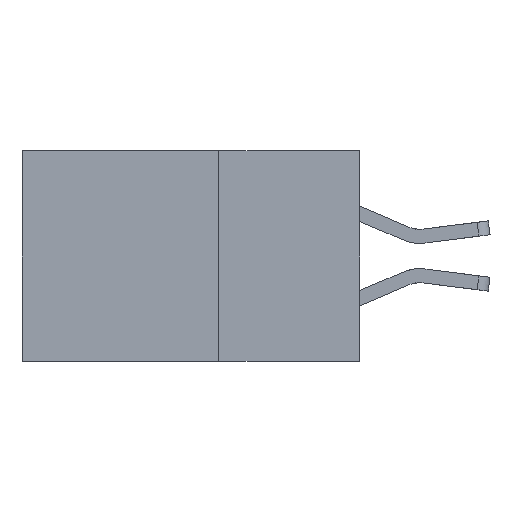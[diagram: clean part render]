
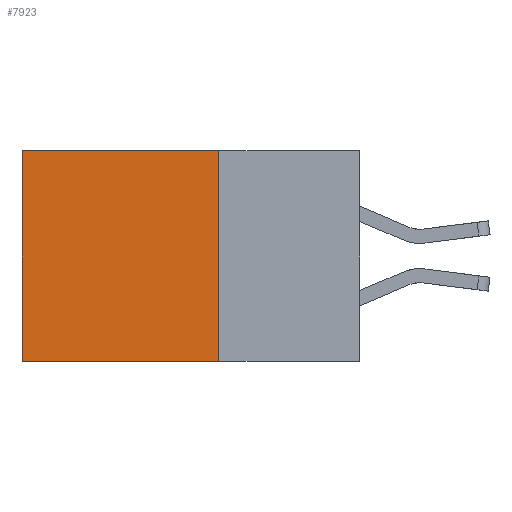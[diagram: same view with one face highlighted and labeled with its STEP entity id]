
A CAD part, left-side view. The second image highlights one B-rep face of the part: STEP entity #7923.
In plain terms, the highlighted planar face has unit normal (-1, 0, 0).
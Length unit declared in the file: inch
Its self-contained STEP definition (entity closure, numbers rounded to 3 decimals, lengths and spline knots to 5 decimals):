
#9 = ORIENTED_EDGE ( 'NONE', *, *, #3762, .F. ) ;
#280 = CARTESIAN_POINT ( 'NONE',  ( 0.2875, 0.25, -0.375 ) ) ;
#349 = CARTESIAN_POINT ( 'NONE',  ( 0.2875, 0.6, -0.375 ) ) ;
#648 = CARTESIAN_POINT ( 'NONE',  ( 0.2875, 0.25, 0. ) ) ;
#745 = VERTEX_POINT ( 'NONE', #4051 ) ;
#1106 = ORIENTED_EDGE ( 'NONE', *, *, #2413, .T. ) ;
#1216 = EDGE_CURVE ( 'NONE', #6039, #4882, #4200, .T. ) ;
#1244 = LINE ( 'NONE', #6938, #5781 ) ;
#1268 = EDGE_LOOP ( 'NONE', ( #1106, #9, #4151, #8144 ) ) ;
#1804 = VECTOR ( 'NONE', #7164, 39.37008 ) ;
#2143 = VECTOR ( 'NONE', #5949, 39.37008 ) ;
#2364 = LINE ( 'NONE', #8767, #2143 ) ;
#2413 = EDGE_CURVE ( 'NONE', #4882, #745, #3729, .T. ) ;
#2790 = CARTESIAN_POINT ( 'NONE',  ( 0.2875, 0.6, 0. ) ) ;
#3080 = DIRECTION ( 'NONE',  ( 1., 0., 0. ) ) ;
#3464 = VECTOR ( 'NONE', #7090, 39.37008 ) ;
#3669 = CARTESIAN_POINT ( 'NONE',  ( 0.2875, 0.25, 0. ) ) ;
#3729 = LINE ( 'NONE', #349, #1804 ) ;
#3762 = EDGE_CURVE ( 'NONE', #4008, #745, #1244, .T. ) ;
#4008 = VERTEX_POINT ( 'NONE', #280 ) ;
#4051 = CARTESIAN_POINT ( 'NONE',  ( 0.2875, 0.6, -0.375 ) ) ;
#4151 = ORIENTED_EDGE ( 'NONE', *, *, #5965, .F. ) ;
#4200 = LINE ( 'NONE', #3669, #3464 ) ;
#4241 = FACE_OUTER_BOUND ( 'NONE', #1268, .T. ) ;
#4479 = CARTESIAN_POINT ( 'NONE',  ( 0.2875, 0.25, -0.375 ) ) ;
#4882 = VERTEX_POINT ( 'NONE', #2790 ) ;
#5781 = VECTOR ( 'NONE', #7034, 39.37008 ) ;
#5949 = DIRECTION ( 'NONE',  ( 0., 0., -1. ) ) ;
#5965 = EDGE_CURVE ( 'NONE', #6039, #4008, #2364, .T. ) ;
#6039 = VERTEX_POINT ( 'NONE', #648 ) ;
#6938 = CARTESIAN_POINT ( 'NONE',  ( 0.2875, 0.25, -0.375 ) ) ;
#7034 = DIRECTION ( 'NONE',  ( 0., 1., 0. ) ) ;
#7090 = DIRECTION ( 'NONE',  ( 0., 1., 0. ) ) ;
#7152 = DIRECTION ( 'NONE',  ( 0., 0., -1. ) ) ;
#7164 = DIRECTION ( 'NONE',  ( 0., 0., -1. ) ) ;
#7282 = AXIS2_PLACEMENT_3D ( 'NONE', #4479, #3080, #7152 ) ;
#7923 = ADVANCED_FACE ( 'NONE', ( #4241 ), #8583, .F. ) ;
#8144 = ORIENTED_EDGE ( 'NONE', *, *, #1216, .T. ) ;
#8583 = PLANE ( 'NONE',  #7282 ) ;
#8767 = CARTESIAN_POINT ( 'NONE',  ( 0.2875, 0.25, -0.375 ) ) ;
